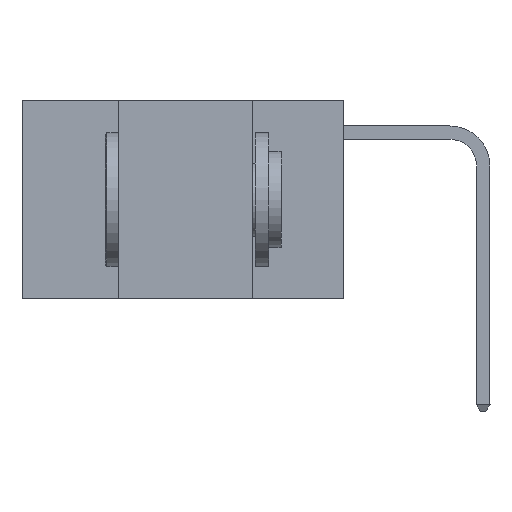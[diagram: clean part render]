
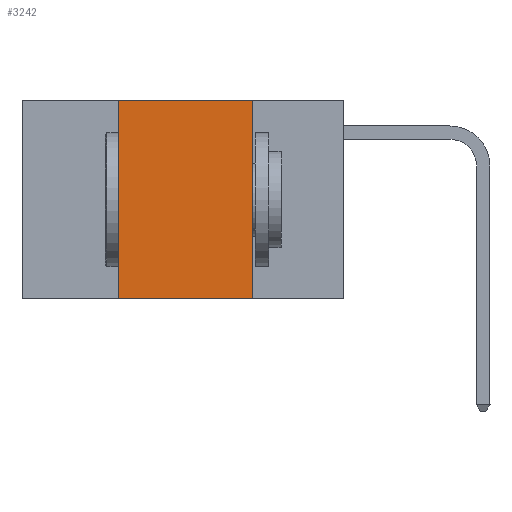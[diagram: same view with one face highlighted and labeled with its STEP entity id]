
A CAD part, left-side view. The second image highlights one B-rep face of the part: STEP entity #3242.
In plain terms, the highlighted planar face has unit normal (-1, 0, 0).
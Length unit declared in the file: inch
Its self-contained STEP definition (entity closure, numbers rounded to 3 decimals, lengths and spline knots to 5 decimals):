
#60 = EDGE_LOOP ( 'NONE', ( #3997, #15784, #10076, #15208 ) ) ;
#1510 = DIRECTION ( 'NONE',  ( 0., 0., -1. ) ) ;
#1688 = DIRECTION ( 'NONE',  ( 1., 0., 0. ) ) ;
#1865 = CARTESIAN_POINT ( 'NONE',  ( 0., 0.17, -0.37 ) ) ;
#2159 = VECTOR ( 'NONE', #13660, 39.37008 ) ;
#3242 = ADVANCED_FACE ( 'NONE', ( #11449 ), #12928, .F. ) ;
#3922 = EDGE_CURVE ( 'NONE', #5787, #9654, #5468, .T. ) ;
#3997 = ORIENTED_EDGE ( 'NONE', *, *, #10656, .F. ) ;
#4781 = LINE ( 'NONE', #14728, #7649 ) ;
#4998 = DIRECTION ( 'NONE',  ( 0., 0., -1. ) ) ;
#5033 = CARTESIAN_POINT ( 'NONE',  ( 0., 0.6, 0. ) ) ;
#5468 = LINE ( 'NONE', #13605, #2159 ) ;
#5787 = VERTEX_POINT ( 'NONE', #10104 ) ;
#6166 = LINE ( 'NONE', #6824, #15541 ) ;
#6824 = CARTESIAN_POINT ( 'NONE',  ( 0., 0.6, 0. ) ) ;
#7347 = LINE ( 'NONE', #14321, #13839 ) ;
#7649 = VECTOR ( 'NONE', #4998, 39.37008 ) ;
#7836 = EDGE_CURVE ( 'NONE', #5787, #11607, #7347, .T. ) ;
#8074 = DIRECTION ( 'NONE',  ( 0., -1., 0. ) ) ;
#8245 = DIRECTION ( 'NONE',  ( 0., -1., 0. ) ) ;
#8391 = EDGE_CURVE ( 'NONE', #9654, #10478, #6166, .T. ) ;
#9654 = VERTEX_POINT ( 'NONE', #11780 ) ;
#10076 = ORIENTED_EDGE ( 'NONE', *, *, #3922, .F. ) ;
#10104 = CARTESIAN_POINT ( 'NONE',  ( 0., 0.42, -0.37 ) ) ;
#10478 = VERTEX_POINT ( 'NONE', #10778 ) ;
#10656 = EDGE_CURVE ( 'NONE', #10478, #11607, #4781, .T. ) ;
#10778 = CARTESIAN_POINT ( 'NONE',  ( 0., 0.17, 0. ) ) ;
#11449 = FACE_OUTER_BOUND ( 'NONE', #60, .T. ) ;
#11595 = AXIS2_PLACEMENT_3D ( 'NONE', #5033, #1688, #1510 ) ;
#11607 = VERTEX_POINT ( 'NONE', #1865 ) ;
#11780 = CARTESIAN_POINT ( 'NONE',  ( 0., 0.42, 0. ) ) ;
#12928 = PLANE ( 'NONE',  #11595 ) ;
#13605 = CARTESIAN_POINT ( 'NONE',  ( 0., 0.42, 0. ) ) ;
#13660 = DIRECTION ( 'NONE',  ( 0., 0., 1. ) ) ;
#13839 = VECTOR ( 'NONE', #8245, 39.37008 ) ;
#14321 = CARTESIAN_POINT ( 'NONE',  ( 0., 0.6, -0.37 ) ) ;
#14728 = CARTESIAN_POINT ( 'NONE',  ( 0., 0.17, 0. ) ) ;
#15208 = ORIENTED_EDGE ( 'NONE', *, *, #7836, .T. ) ;
#15541 = VECTOR ( 'NONE', #8074, 39.37008 ) ;
#15784 = ORIENTED_EDGE ( 'NONE', *, *, #8391, .F. ) ;
